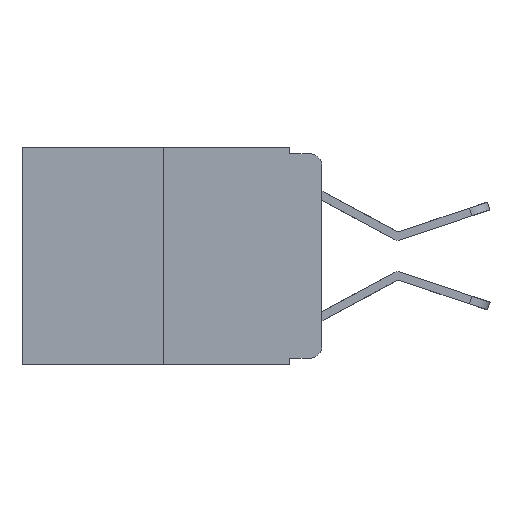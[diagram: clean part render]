
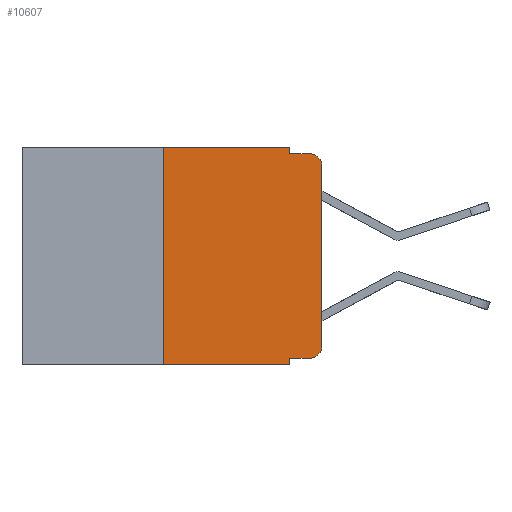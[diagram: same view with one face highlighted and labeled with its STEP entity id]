
A CAD part, left-side view. The second image highlights one B-rep face of the part: STEP entity #10607.
In plain terms, the highlighted planar face has unit normal (-1, 0, 0).
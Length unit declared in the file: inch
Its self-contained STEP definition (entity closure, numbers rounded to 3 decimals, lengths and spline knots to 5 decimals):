
#110 = ORIENTED_EDGE ( 'NONE', *, *, #16485, .T. ) ;
#281 = ORIENTED_EDGE ( 'NONE', *, *, #8428, .F. ) ;
#317 = ORIENTED_EDGE ( 'NONE', *, *, #1205, .F. ) ;
#558 = VERTEX_POINT ( 'NONE', #14509 ) ;
#901 = CARTESIAN_POINT ( 'NONE',  ( 0., 0.473, 0. ) ) ;
#1205 = EDGE_CURVE ( 'NONE', #23470, #12203, #10093, .T. ) ;
#1913 = CARTESIAN_POINT ( 'NONE',  ( 0., 0.051, -0.333 ) ) ;
#1914 = DIRECTION ( 'NONE',  ( 0., 0., 1. ) ) ;
#2031 = VECTOR ( 'NONE', #6829, 39.37008 ) ;
#2714 = DIRECTION ( 'NONE',  ( 0., -1., 0. ) ) ;
#3002 = EDGE_CURVE ( 'NONE', #16252, #12575, #14431, .T. ) ;
#3144 = VECTOR ( 'NONE', #14035, 39.37008 ) ;
#3658 = ORIENTED_EDGE ( 'NONE', *, *, #3002, .T. ) ;
#4326 = VECTOR ( 'NONE', #2714, 39.37008 ) ;
#5106 = CARTESIAN_POINT ( 'NONE',  ( 0., 0.25, 0. ) ) ;
#5337 = VECTOR ( 'NONE', #1914, 39.37008 ) ;
#5701 = LINE ( 'NONE', #16434, #23682 ) ;
#6514 = ORIENTED_EDGE ( 'NONE', *, *, #19018, .F. ) ;
#6829 = DIRECTION ( 'NONE',  ( 0., -1., 0. ) ) ;
#7615 = EDGE_CURVE ( 'NONE', #9251, #22543, #10752, .T. ) ;
#8298 = PLANE ( 'NONE',  #12880 ) ;
#8428 = EDGE_CURVE ( 'NONE', #22776, #22095, #8496, .T. ) ;
#8496 = LINE ( 'NONE', #10200, #2031 ) ;
#8787 = EDGE_CURVE ( 'NONE', #9251, #12203, #20996, .T. ) ;
#9251 = VERTEX_POINT ( 'NONE', #19318 ) ;
#9508 = CARTESIAN_POINT ( 'NONE',  ( 0., 0., -0.313 ) ) ;
#9746 = DIRECTION ( 'NONE',  ( 0., 0., -1. ) ) ;
#10093 = LINE ( 'NONE', #13852, #20946 ) ;
#10200 = CARTESIAN_POINT ( 'NONE',  ( 0., 0.051, -0.01 ) ) ;
#10351 = VECTOR ( 'NONE', #15522, 39.37008 ) ;
#10607 = ADVANCED_FACE ( 'NONE', ( #17379 ), #8298, .F. ) ;
#10752 = LINE ( 'NONE', #5106, #3144 ) ;
#11024 = CARTESIAN_POINT ( 'NONE',  ( 0., 0., 0. ) ) ;
#11094 = AXIS2_PLACEMENT_3D ( 'NONE', #14233, #21789, #22032 ) ;
#11359 = VECTOR ( 'NONE', #13223, 39.37008 ) ;
#11373 = EDGE_LOOP ( 'NONE', ( #3658, #110, #281, #6514, #21150, #14982, #23169, #317, #16683, #21534 ) ) ;
#11483 = AXIS2_PLACEMENT_3D ( 'NONE', #15663, #13401, #9746 ) ;
#11561 = CARTESIAN_POINT ( 'NONE',  ( 0., 0.051, -0.343 ) ) ;
#11827 = EDGE_CURVE ( 'NONE', #23470, #558, #14657, .T. ) ;
#11907 = DIRECTION ( 'NONE',  ( 0., 0., -1. ) ) ;
#12203 = VERTEX_POINT ( 'NONE', #11561 ) ;
#12575 = VERTEX_POINT ( 'NONE', #12895 ) ;
#12880 = AXIS2_PLACEMENT_3D ( 'NONE', #901, #19090, #15683 ) ;
#12895 = CARTESIAN_POINT ( 'NONE',  ( 0., 0., -0.03 ) ) ;
#12996 = EDGE_CURVE ( 'NONE', #22543, #23105, #5701, .T. ) ;
#13223 = DIRECTION ( 'NONE',  ( 0., -1., 0. ) ) ;
#13401 = DIRECTION ( 'NONE',  ( -1., 0., 0. ) ) ;
#13852 = CARTESIAN_POINT ( 'NONE',  ( 0., 0.051, 0. ) ) ;
#14035 = DIRECTION ( 'NONE',  ( 0., 0., 1. ) ) ;
#14233 = CARTESIAN_POINT ( 'NONE',  ( 0., 0.02, -0.03 ) ) ;
#14431 = LINE ( 'NONE', #11024, #5337 ) ;
#14509 = CARTESIAN_POINT ( 'NONE',  ( 0., 0.02, -0.333 ) ) ;
#14657 = LINE ( 'NONE', #1913, #11359 ) ;
#14982 = ORIENTED_EDGE ( 'NONE', *, *, #7615, .F. ) ;
#15522 = DIRECTION ( 'NONE',  ( 0., 0., -1. ) ) ;
#15546 = CARTESIAN_POINT ( 'NONE',  ( 0., 0.051, -0.333 ) ) ;
#15663 = CARTESIAN_POINT ( 'NONE',  ( 0., 0.02, -0.313 ) ) ;
#15683 = DIRECTION ( 'NONE',  ( 0., 0., -1. ) ) ;
#15814 = CARTESIAN_POINT ( 'NONE',  ( 0., 0.051, 0. ) ) ;
#16252 = VERTEX_POINT ( 'NONE', #9508 ) ;
#16434 = CARTESIAN_POINT ( 'NONE',  ( 0., 0.473, 0. ) ) ;
#16485 = EDGE_CURVE ( 'NONE', #12575, #22095, #18051, .T. ) ;
#16683 = ORIENTED_EDGE ( 'NONE', *, *, #11827, .T. ) ;
#16882 = CIRCLE ( 'NONE', #11483, 0.02 ) ;
#17379 = FACE_OUTER_BOUND ( 'NONE', #11373, .T. ) ;
#18051 = CIRCLE ( 'NONE', #11094, 0.02 ) ;
#18532 = EDGE_CURVE ( 'NONE', #558, #16252, #16882, .T. ) ;
#18936 = CARTESIAN_POINT ( 'NONE',  ( 0., 0.02, -0.01 ) ) ;
#19018 = EDGE_CURVE ( 'NONE', #23105, #22776, #19147, .T. ) ;
#19090 = DIRECTION ( 'NONE',  ( 1., 0., 0. ) ) ;
#19147 = LINE ( 'NONE', #19265, #10351 ) ;
#19265 = CARTESIAN_POINT ( 'NONE',  ( 0., 0.051, 0. ) ) ;
#19318 = CARTESIAN_POINT ( 'NONE',  ( 0., 0.25, -0.343 ) ) ;
#20055 = CARTESIAN_POINT ( 'NONE',  ( 0., 0.051, -0.01 ) ) ;
#20946 = VECTOR ( 'NONE', #11907, 39.37008 ) ;
#20996 = LINE ( 'NONE', #21121, #4326 ) ;
#21121 = CARTESIAN_POINT ( 'NONE',  ( 0., 0.473, -0.343 ) ) ;
#21150 = ORIENTED_EDGE ( 'NONE', *, *, #12996, .F. ) ;
#21534 = ORIENTED_EDGE ( 'NONE', *, *, #18532, .T. ) ;
#21729 = DIRECTION ( 'NONE',  ( 0., -1., 0. ) ) ;
#21789 = DIRECTION ( 'NONE',  ( -1., 0., 0. ) ) ;
#22032 = DIRECTION ( 'NONE',  ( 0., 0., -1. ) ) ;
#22095 = VERTEX_POINT ( 'NONE', #18936 ) ;
#22543 = VERTEX_POINT ( 'NONE', #23309 ) ;
#22776 = VERTEX_POINT ( 'NONE', #20055 ) ;
#23105 = VERTEX_POINT ( 'NONE', #15814 ) ;
#23169 = ORIENTED_EDGE ( 'NONE', *, *, #8787, .T. ) ;
#23309 = CARTESIAN_POINT ( 'NONE',  ( 0., 0.25, 0. ) ) ;
#23470 = VERTEX_POINT ( 'NONE', #15546 ) ;
#23682 = VECTOR ( 'NONE', #21729, 39.37008 ) ;
